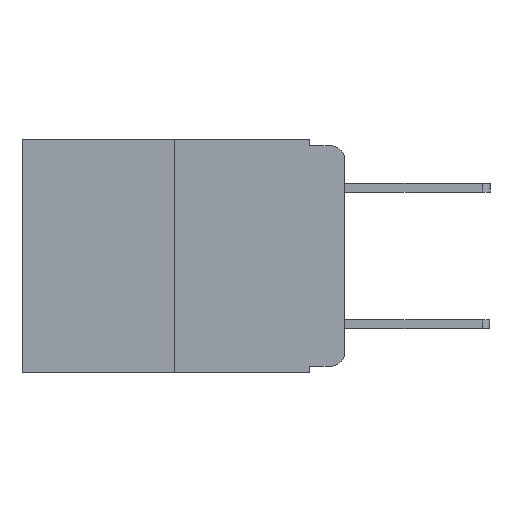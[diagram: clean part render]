
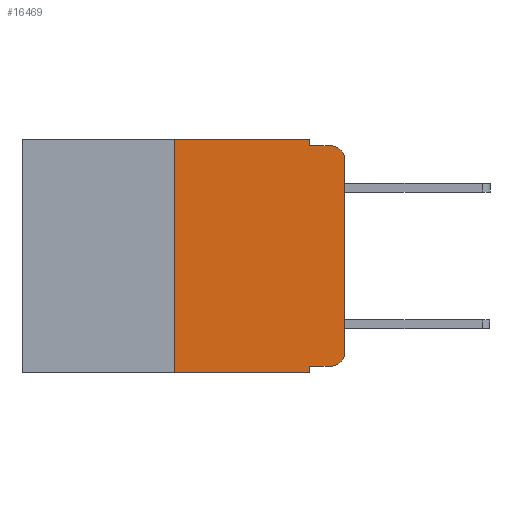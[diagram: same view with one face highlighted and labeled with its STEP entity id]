
A CAD part, left-side view. The second image highlights one B-rep face of the part: STEP entity #16469.
In plain terms, the highlighted planar face has unit normal (-1, 0, 0).
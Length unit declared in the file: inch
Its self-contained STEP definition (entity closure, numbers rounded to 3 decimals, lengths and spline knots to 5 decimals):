
#420 = EDGE_CURVE ( 'NONE', #15603, #1734, #6824, .T. ) ;
#514 = VERTEX_POINT ( 'NONE', #11679 ) ;
#785 = DIRECTION ( 'NONE',  ( -1., 0., 0. ) ) ;
#847 = PLANE ( 'NONE',  #21100 ) ;
#1169 = LINE ( 'NONE', #18555, #10007 ) ;
#1582 = EDGE_LOOP ( 'NONE', ( #5343, #9935, #1647, #13147, #13712, #18779, #5634, #3108, #3666, #17761 ) ) ;
#1647 = ORIENTED_EDGE ( 'NONE', *, *, #4078, .F. ) ;
#1734 = VERTEX_POINT ( 'NONE', #3856 ) ;
#1847 = DIRECTION ( 'NONE',  ( 0., 0., 1. ) ) ;
#3044 = LINE ( 'NONE', #14149, #7767 ) ;
#3108 = ORIENTED_EDGE ( 'NONE', *, *, #16283, .F. ) ;
#3187 = AXIS2_PLACEMENT_3D ( 'NONE', #6362, #18370, #8130 ) ;
#3332 = VERTEX_POINT ( 'NONE', #5846 ) ;
#3512 = VERTEX_POINT ( 'NONE', #6068 ) ;
#3666 = ORIENTED_EDGE ( 'NONE', *, *, #17244, .T. ) ;
#3856 = CARTESIAN_POINT ( 'NONE',  ( 0., 0.25, 0. ) ) ;
#4039 = CARTESIAN_POINT ( 'NONE',  ( 0., 0.051, 0. ) ) ;
#4078 = EDGE_CURVE ( 'NONE', #16744, #3332, #3044, .T. ) ;
#4415 = CARTESIAN_POINT ( 'NONE',  ( 0., 0.473, 0. ) ) ;
#4903 = CARTESIAN_POINT ( 'NONE',  ( 0., 0.051, -0.343 ) ) ;
#5343 = ORIENTED_EDGE ( 'NONE', *, *, #5571, .T. ) ;
#5571 = EDGE_CURVE ( 'NONE', #12190, #18663, #6584, .T. ) ;
#5634 = ORIENTED_EDGE ( 'NONE', *, *, #15848, .T. ) ;
#5833 = DIRECTION ( 'NONE',  ( 0., 0., -1. ) ) ;
#5846 = CARTESIAN_POINT ( 'NONE',  ( 0., 0.02, -0.01 ) ) ;
#5869 = LINE ( 'NONE', #16875, #14529 ) ;
#5872 = EDGE_CURVE ( 'NONE', #1734, #10474, #1169, .T. ) ;
#6068 = CARTESIAN_POINT ( 'NONE',  ( 0., 0.02, -0.333 ) ) ;
#6362 = CARTESIAN_POINT ( 'NONE',  ( 0., 0.02, -0.313 ) ) ;
#6584 = LINE ( 'NONE', #9897, #15258 ) ;
#6824 = LINE ( 'NONE', #21735, #14951 ) ;
#6899 = EDGE_CURVE ( 'NONE', #18663, #3332, #16223, .T. ) ;
#7767 = VECTOR ( 'NONE', #19853, 39.37008 ) ;
#8061 = DIRECTION ( 'NONE',  ( 0., -1., 0. ) ) ;
#8130 = DIRECTION ( 'NONE',  ( 0., 0., -1. ) ) ;
#8675 = VECTOR ( 'NONE', #17789, 39.37008 ) ;
#8698 = VECTOR ( 'NONE', #8061, 39.37008 ) ;
#9743 = DIRECTION ( 'NONE',  ( 0., 0., -1. ) ) ;
#9897 = CARTESIAN_POINT ( 'NONE',  ( 0., 0., 0. ) ) ;
#9935 = ORIENTED_EDGE ( 'NONE', *, *, #6899, .T. ) ;
#10007 = VECTOR ( 'NONE', #15191, 39.37008 ) ;
#10268 = DIRECTION ( 'NONE',  ( 0., 0., 1. ) ) ;
#10474 = VERTEX_POINT ( 'NONE', #18277 ) ;
#11334 = CARTESIAN_POINT ( 'NONE',  ( 0., 0.02, -0.03 ) ) ;
#11679 = CARTESIAN_POINT ( 'NONE',  ( 0., 0.051, -0.333 ) ) ;
#12190 = VERTEX_POINT ( 'NONE', #13138 ) ;
#12795 = CARTESIAN_POINT ( 'NONE',  ( 0., 0., -0.03 ) ) ;
#13056 = DIRECTION ( 'NONE',  ( 0., 0., -1. ) ) ;
#13138 = CARTESIAN_POINT ( 'NONE',  ( 0., 0., -0.313 ) ) ;
#13147 = ORIENTED_EDGE ( 'NONE', *, *, #19778, .F. ) ;
#13196 = LINE ( 'NONE', #14932, #8698 ) ;
#13452 = FACE_OUTER_BOUND ( 'NONE', #1582, .T. ) ;
#13683 = VECTOR ( 'NONE', #5833, 39.37008 ) ;
#13712 = ORIENTED_EDGE ( 'NONE', *, *, #5872, .F. ) ;
#14149 = CARTESIAN_POINT ( 'NONE',  ( 0., 0.051, -0.01 ) ) ;
#14246 = CARTESIAN_POINT ( 'NONE',  ( 0., 0.25, -0.343 ) ) ;
#14250 = LINE ( 'NONE', #4039, #13683 ) ;
#14529 = VECTOR ( 'NONE', #18546, 39.37008 ) ;
#14932 = CARTESIAN_POINT ( 'NONE',  ( 0., 0.473, -0.343 ) ) ;
#14951 = VECTOR ( 'NONE', #1847, 39.37008 ) ;
#15191 = DIRECTION ( 'NONE',  ( 0., -1., 0. ) ) ;
#15258 = VECTOR ( 'NONE', #10268, 39.37008 ) ;
#15603 = VERTEX_POINT ( 'NONE', #14246 ) ;
#15848 = EDGE_CURVE ( 'NONE', #15603, #20880, #13196, .T. ) ;
#16112 = CARTESIAN_POINT ( 'NONE',  ( 0., 0.051, 0. ) ) ;
#16223 = CIRCLE ( 'NONE', #17111, 0.02 ) ;
#16283 = EDGE_CURVE ( 'NONE', #514, #20880, #22143, .T. ) ;
#16469 = ADVANCED_FACE ( 'NONE', ( #13452 ), #847, .F. ) ;
#16744 = VERTEX_POINT ( 'NONE', #20593 ) ;
#16875 = CARTESIAN_POINT ( 'NONE',  ( 0., 0.051, -0.333 ) ) ;
#17111 = AXIS2_PLACEMENT_3D ( 'NONE', #11334, #785, #13056 ) ;
#17244 = EDGE_CURVE ( 'NONE', #514, #3512, #5869, .T. ) ;
#17761 = ORIENTED_EDGE ( 'NONE', *, *, #20767, .T. ) ;
#17789 = DIRECTION ( 'NONE',  ( 0., 0., -1. ) ) ;
#18277 = CARTESIAN_POINT ( 'NONE',  ( 0., 0.051, 0. ) ) ;
#18370 = DIRECTION ( 'NONE',  ( -1., 0., 0. ) ) ;
#18546 = DIRECTION ( 'NONE',  ( 0., -1., 0. ) ) ;
#18555 = CARTESIAN_POINT ( 'NONE',  ( 0., 0.473, 0. ) ) ;
#18663 = VERTEX_POINT ( 'NONE', #12795 ) ;
#18779 = ORIENTED_EDGE ( 'NONE', *, *, #420, .F. ) ;
#19470 = CIRCLE ( 'NONE', #3187, 0.02 ) ;
#19778 = EDGE_CURVE ( 'NONE', #10474, #16744, #14250, .T. ) ;
#19853 = DIRECTION ( 'NONE',  ( 0., -1., 0. ) ) ;
#19938 = DIRECTION ( 'NONE',  ( 1., 0., 0. ) ) ;
#20593 = CARTESIAN_POINT ( 'NONE',  ( 0., 0.051, -0.01 ) ) ;
#20767 = EDGE_CURVE ( 'NONE', #3512, #12190, #19470, .T. ) ;
#20880 = VERTEX_POINT ( 'NONE', #4903 ) ;
#21100 = AXIS2_PLACEMENT_3D ( 'NONE', #4415, #19938, #9743 ) ;
#21735 = CARTESIAN_POINT ( 'NONE',  ( 0., 0.25, 0. ) ) ;
#22143 = LINE ( 'NONE', #16112, #8675 ) ;
